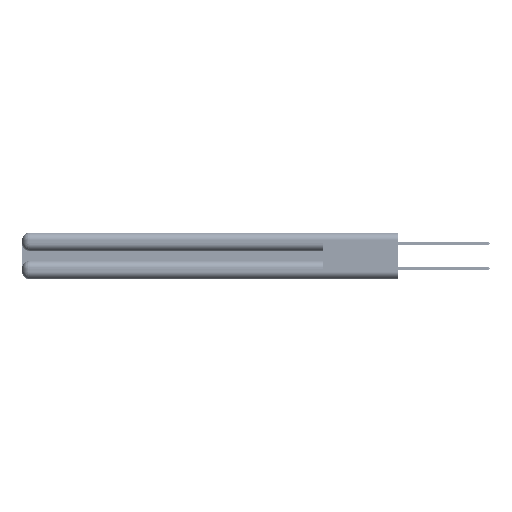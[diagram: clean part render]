
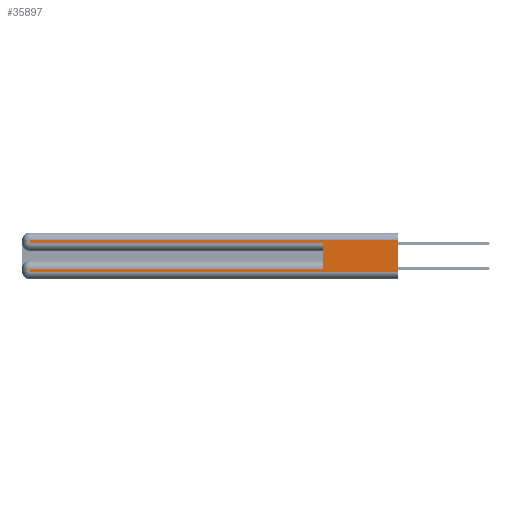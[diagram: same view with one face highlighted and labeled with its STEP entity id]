
A CAD part, left-side view. The second image highlights one B-rep face of the part: STEP entity #35897.
In plain terms, the highlighted planar face has unit normal (-1, 0, 0).
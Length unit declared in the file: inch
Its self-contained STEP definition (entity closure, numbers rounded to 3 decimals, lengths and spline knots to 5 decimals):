
#52 = VERTEX_POINT ( 'NONE', #26045 ) ;
#853 = ORIENTED_EDGE ( 'NONE', *, *, #4636, .T. ) ;
#1766 = VECTOR ( 'NONE', #30275, 39.37008 ) ;
#2578 = CARTESIAN_POINT ( 'NONE',  ( 0., 0.6, 0.085 ) ) ;
#3397 = CARTESIAN_POINT ( 'NONE',  ( 0., 0., 0.06 ) ) ;
#3727 = DIRECTION ( 'NONE',  ( 0., -1., 0. ) ) ;
#3947 = DIRECTION ( 'NONE',  ( 0., 1., 0. ) ) ;
#3966 = VECTOR ( 'NONE', #17533, 39.37008 ) ;
#4636 = EDGE_CURVE ( 'NONE', #46348, #44282, #19924, .T. ) ;
#5364 = DIRECTION ( 'NONE',  ( 0., 0., -1. ) ) ;
#7078 = EDGE_CURVE ( 'NONE', #51070, #46348, #33487, .T. ) ;
#7236 = DIRECTION ( 'NONE',  ( 0., 0., 1. ) ) ;
#8404 = DIRECTION ( 'NONE',  ( 1., 0., 0. ) ) ;
#8503 = LINE ( 'NONE', #10057, #30819 ) ;
#9188 = FACE_OUTER_BOUND ( 'NONE', #30178, .T. ) ;
#10057 = CARTESIAN_POINT ( 'NONE',  ( 0., 0., 0.31 ) ) ;
#11913 = ORIENTED_EDGE ( 'NONE', *, *, #49889, .T. ) ;
#12645 = PLANE ( 'NONE',  #15502 ) ;
#13320 = CARTESIAN_POINT ( 'NONE',  ( 0., 2.94, 0.37 ) ) ;
#15502 = AXIS2_PLACEMENT_3D ( 'NONE', #52843, #8404, #39556 ) ;
#16719 = LINE ( 'NONE', #38204, #50903 ) ;
#17533 = DIRECTION ( 'NONE',  ( 0., 0., -1. ) ) ;
#18987 = DIRECTION ( 'NONE',  ( 0., 1., 0. ) ) ;
#19924 = LINE ( 'NONE', #30417, #45033 ) ;
#20231 = VECTOR ( 'NONE', #41444, 39.37008 ) ;
#21173 = EDGE_CURVE ( 'NONE', #57618, #44282, #16719, .T. ) ;
#23215 = EDGE_CURVE ( 'NONE', #52, #31050, #51366, .T. ) ;
#25447 = LINE ( 'NONE', #3397, #1766 ) ;
#26045 = CARTESIAN_POINT ( 'NONE',  ( 0., 0., 0.31 ) ) ;
#26424 = VERTEX_POINT ( 'NONE', #52304 ) ;
#27165 = ORIENTED_EDGE ( 'NONE', *, *, #21173, .F. ) ;
#27235 = ORIENTED_EDGE ( 'NONE', *, *, #43214, .T. ) ;
#29162 = CARTESIAN_POINT ( 'NONE',  ( 0., 2.94, 0.285 ) ) ;
#30178 = EDGE_LOOP ( 'NONE', ( #44099, #35605, #43368, #853, #27165, #11913, #27235, #46493 ) ) ;
#30275 = DIRECTION ( 'NONE',  ( 0., -1., 0. ) ) ;
#30417 = CARTESIAN_POINT ( 'NONE',  ( 0., 0., 0.285 ) ) ;
#30637 = CARTESIAN_POINT ( 'NONE',  ( 0., 0., 0.085 ) ) ;
#30819 = VECTOR ( 'NONE', #18987, 39.37008 ) ;
#31050 = VERTEX_POINT ( 'NONE', #36081 ) ;
#33487 = LINE ( 'NONE', #36985, #20231 ) ;
#35605 = ORIENTED_EDGE ( 'NONE', *, *, #55503, .T. ) ;
#35897 = ADVANCED_FACE ( 'NONE', ( #9188 ), #12645, .F. ) ;
#36081 = CARTESIAN_POINT ( 'NONE',  ( 0., 0., 0.06 ) ) ;
#36985 = CARTESIAN_POINT ( 'NONE',  ( 0., 2.94, 0.37 ) ) ;
#37109 = LINE ( 'NONE', #13320, #46163 ) ;
#37347 = CARTESIAN_POINT ( 'NONE',  ( 0., 2.94, 0.06 ) ) ;
#37524 = VECTOR ( 'NONE', #3947, 39.37008 ) ;
#38204 = CARTESIAN_POINT ( 'NONE',  ( 0., 0.6, 0.145 ) ) ;
#38902 = VERTEX_POINT ( 'NONE', #37347 ) ;
#38934 = LINE ( 'NONE', #30637, #37524 ) ;
#39556 = DIRECTION ( 'NONE',  ( 0., 0., -1. ) ) ;
#39758 = CARTESIAN_POINT ( 'NONE',  ( 0., 0., 0.37 ) ) ;
#41444 = DIRECTION ( 'NONE',  ( 0., 0., -1. ) ) ;
#41819 = EDGE_CURVE ( 'NONE', #38902, #31050, #25447, .T. ) ;
#43214 = EDGE_CURVE ( 'NONE', #26424, #38902, #37109, .T. ) ;
#43368 = ORIENTED_EDGE ( 'NONE', *, *, #7078, .T. ) ;
#44099 = ORIENTED_EDGE ( 'NONE', *, *, #23215, .F. ) ;
#44282 = VERTEX_POINT ( 'NONE', #51641 ) ;
#45033 = VECTOR ( 'NONE', #3727, 39.37008 ) ;
#46163 = VECTOR ( 'NONE', #5364, 39.37008 ) ;
#46348 = VERTEX_POINT ( 'NONE', #29162 ) ;
#46493 = ORIENTED_EDGE ( 'NONE', *, *, #41819, .T. ) ;
#46791 = CARTESIAN_POINT ( 'NONE',  ( 0., 2.94, 0.31 ) ) ;
#49889 = EDGE_CURVE ( 'NONE', #57618, #26424, #38934, .T. ) ;
#50903 = VECTOR ( 'NONE', #7236, 39.37008 ) ;
#51070 = VERTEX_POINT ( 'NONE', #46791 ) ;
#51366 = LINE ( 'NONE', #39758, #3966 ) ;
#51641 = CARTESIAN_POINT ( 'NONE',  ( 0., 0.6, 0.285 ) ) ;
#52304 = CARTESIAN_POINT ( 'NONE',  ( 0., 2.94, 0.085 ) ) ;
#52843 = CARTESIAN_POINT ( 'NONE',  ( 0., 0., 0.37 ) ) ;
#55503 = EDGE_CURVE ( 'NONE', #52, #51070, #8503, .T. ) ;
#57618 = VERTEX_POINT ( 'NONE', #2578 ) ;
